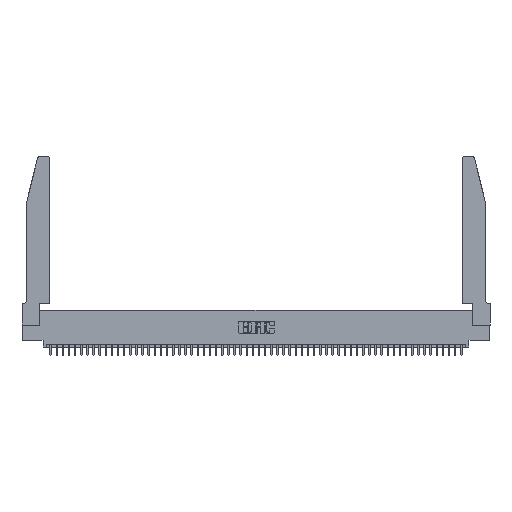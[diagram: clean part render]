
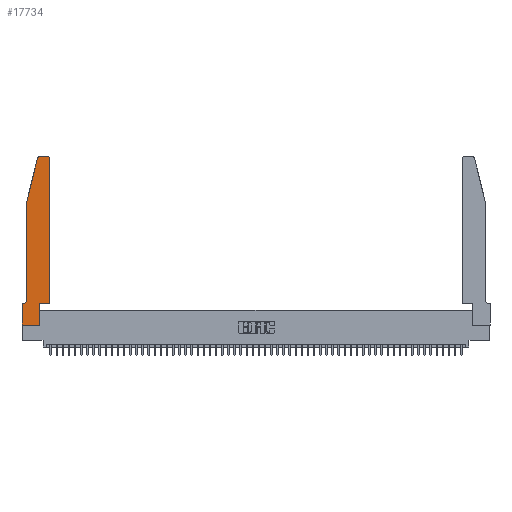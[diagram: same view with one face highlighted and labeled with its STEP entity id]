
A CAD part, top view. The second image highlights one B-rep face of the part: STEP entity #17734.
In plain terms, the highlighted planar face has unit normal (0, 0, 1).
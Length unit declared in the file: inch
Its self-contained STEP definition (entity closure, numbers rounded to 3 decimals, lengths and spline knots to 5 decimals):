
#117 = VERTEX_POINT ( 'NONE', #24283 ) ;
#540 = LINE ( 'NONE', #28226, #33080 ) ;
#622 = DIRECTION ( 'NONE',  ( 1., 0., 0. ) ) ;
#1321 = LINE ( 'NONE', #30457, #33818 ) ;
#1773 = DIRECTION ( 'NONE',  ( 0., 1., 0. ) ) ;
#2243 = CARTESIAN_POINT ( 'NONE',  ( 0.2865, 0.35, 0.37 ) ) ;
#3311 = VERTEX_POINT ( 'NONE', #41952 ) ;
#4764 = AXIS2_PLACEMENT_3D ( 'NONE', #52568, #23818, #53309 ) ;
#4837 = ORIENTED_EDGE ( 'NONE', *, *, #7785, .T. ) ;
#6080 = ORIENTED_EDGE ( 'NONE', *, *, #40368, .T. ) ;
#6818 = EDGE_CURVE ( 'NONE', #35872, #3311, #26489, .T. ) ;
#7785 = EDGE_CURVE ( 'NONE', #3311, #49695, #48779, .T. ) ;
#7859 = VERTEX_POINT ( 'NONE', #28221 ) ;
#7978 = DIRECTION ( 'NONE',  ( 0., 0., 1. ) ) ;
#9416 = ORIENTED_EDGE ( 'NONE', *, *, #14255, .T. ) ;
#9960 = EDGE_CURVE ( 'NONE', #49695, #24837, #51154, .T. ) ;
#10256 = PLANE ( 'NONE',  #4764 ) ;
#10703 = CIRCLE ( 'NONE', #19130, 0.03 ) ;
#10855 = AXIS2_PLACEMENT_3D ( 'NONE', #48891, #23642, #53141 ) ;
#11014 = CARTESIAN_POINT ( 'NONE',  ( 0.4505, 0.35, 0.37 ) ) ;
#11652 = VERTEX_POINT ( 'NONE', #25148 ) ;
#12089 = ORIENTED_EDGE ( 'NONE', *, *, #32029, .T. ) ;
#13085 = CARTESIAN_POINT ( 'NONE',  ( 0.0055, 0.42, 0.37 ) ) ;
#13315 = CARTESIAN_POINT ( 'NONE',  ( 0.4505, 2.72, 0.37 ) ) ;
#14255 = EDGE_CURVE ( 'NONE', #52962, #23506, #51151, .T. ) ;
#15231 = VECTOR ( 'NONE', #622, 39.37008 ) ;
#16194 = VECTOR ( 'NONE', #20317, 39.37008 ) ;
#16230 = CARTESIAN_POINT ( 'NONE',  ( 0.0755, 0.35, 0.37 ) ) ;
#17378 = DIRECTION ( 'NONE',  ( -1., 0., 0. ) ) ;
#17525 = VECTOR ( 'NONE', #19637, 39.37008 ) ;
#17734 = ADVANCED_FACE ( 'NONE', ( #28120 ), #10256, .T. ) ;
#18109 = ORIENTED_EDGE ( 'NONE', *, *, #43499, .T. ) ;
#18536 = CARTESIAN_POINT ( 'NONE',  ( 0.0755, 2., 0.37 ) ) ;
#18870 = VECTOR ( 'NONE', #25044, 39.37008 ) ;
#19130 = AXIS2_PLACEMENT_3D ( 'NONE', #33383, #7978, #37609 ) ;
#19637 = DIRECTION ( 'NONE',  ( 1., 0., 0. ) ) ;
#20111 = ORIENTED_EDGE ( 'NONE', *, *, #31610, .T. ) ;
#20317 = DIRECTION ( 'NONE',  ( -1., 0., 0. ) ) ;
#20764 = CARTESIAN_POINT ( 'NONE',  ( 0.25487, 2.72718, 0.37 ) ) ;
#21594 = CARTESIAN_POINT ( 'NONE',  ( 0., 0., 0.37 ) ) ;
#21973 = DIRECTION ( 'NONE',  ( 0., -1., 0. ) ) ;
#23506 = VERTEX_POINT ( 'NONE', #40249 ) ;
#23642 = DIRECTION ( 'NONE',  ( 0., 0., 1. ) ) ;
#23717 = VECTOR ( 'NONE', #40360, 39.37008 ) ;
#23818 = DIRECTION ( 'NONE',  ( 0., 0., 1. ) ) ;
#24283 = CARTESIAN_POINT ( 'NONE',  ( 0.284, 2.75, 0.37 ) ) ;
#24837 = VERTEX_POINT ( 'NONE', #32240 ) ;
#25044 = DIRECTION ( 'NONE',  ( 0., -1., 0. ) ) ;
#25148 = CARTESIAN_POINT ( 'NONE',  ( 0.0755, 0.42, 0.37 ) ) ;
#26302 = EDGE_CURVE ( 'NONE', #7859, #117, #540, .T. ) ;
#26489 = LINE ( 'NONE', #51314, #15231 ) ;
#26869 = CIRCLE ( 'NONE', #45043, 0.07 ) ;
#27215 = CARTESIAN_POINT ( 'NONE',  ( 0.4505, 0.35, 0.37 ) ) ;
#28120 = FACE_OUTER_BOUND ( 'NONE', #33603, .T. ) ;
#28221 = CARTESIAN_POINT ( 'NONE',  ( 0.4205, 2.75, 0.37 ) ) ;
#28226 = CARTESIAN_POINT ( 'NONE',  ( 0.2605, 2.75, 0.37 ) ) ;
#30098 = LINE ( 'NONE', #41820, #18870 ) ;
#30457 = CARTESIAN_POINT ( 'NONE',  ( 0., 0., 0.37 ) ) ;
#31186 = CARTESIAN_POINT ( 'NONE',  ( 0.0055, 0.35, 0.37 ) ) ;
#31558 = VERTEX_POINT ( 'NONE', #18536 ) ;
#31610 = EDGE_CURVE ( 'NONE', #24837, #47314, #39236, .T. ) ;
#32029 = EDGE_CURVE ( 'NONE', #39002, #31558, #43125, .T. ) ;
#32240 = CARTESIAN_POINT ( 'NONE',  ( 0.4505, 0.35, 0.37 ) ) ;
#32929 = ORIENTED_EDGE ( 'NONE', *, *, #48610, .T. ) ;
#33080 = VECTOR ( 'NONE', #53614, 39.37008 ) ;
#33383 = CARTESIAN_POINT ( 'NONE',  ( 0.4205, 2.72, 0.37 ) ) ;
#33424 = ORIENTED_EDGE ( 'NONE', *, *, #44483, .T. ) ;
#33603 = EDGE_LOOP ( 'NONE', ( #45019, #18109, #12089, #6080, #32929, #9416, #34873, #53192, #4837, #44363, #20111, #33424 ) ) ;
#33818 = VECTOR ( 'NONE', #21973, 39.37008 ) ;
#34873 = ORIENTED_EDGE ( 'NONE', *, *, #52831, .T. ) ;
#35872 = VERTEX_POINT ( 'NONE', #21594 ) ;
#36809 = CARTESIAN_POINT ( 'NONE',  ( 0.2865, 0.35, 0.37 ) ) ;
#37609 = DIRECTION ( 'NONE',  ( 1., 0., 0. ) ) ;
#39002 = VERTEX_POINT ( 'NONE', #20764 ) ;
#39236 = LINE ( 'NONE', #27215, #50412 ) ;
#40249 = CARTESIAN_POINT ( 'NONE',  ( 0., 0.35, 0.37 ) ) ;
#40360 = DIRECTION ( 'NONE',  ( 0., 1., 0. ) ) ;
#40368 = EDGE_CURVE ( 'NONE', #31558, #11652, #30098, .T. ) ;
#40534 = CIRCLE ( 'NONE', #10855, 0.03 ) ;
#41820 = CARTESIAN_POINT ( 'NONE',  ( 0.0755, 2., 0.37 ) ) ;
#41952 = CARTESIAN_POINT ( 'NONE',  ( 0.2865, 0., 0.37 ) ) ;
#42638 = DIRECTION ( 'NONE',  ( 0., 0., -1. ) ) ;
#43125 = LINE ( 'NONE', #46692, #51690 ) ;
#43499 = EDGE_CURVE ( 'NONE', #117, #39002, #40534, .T. ) ;
#44363 = ORIENTED_EDGE ( 'NONE', *, *, #9960, .T. ) ;
#44483 = EDGE_CURVE ( 'NONE', #47314, #7859, #10703, .T. ) ;
#45019 = ORIENTED_EDGE ( 'NONE', *, *, #26302, .T. ) ;
#45043 = AXIS2_PLACEMENT_3D ( 'NONE', #13085, #42638, #17378 ) ;
#46692 = CARTESIAN_POINT ( 'NONE',  ( 0.0755, 2., 0.37 ) ) ;
#47314 = VERTEX_POINT ( 'NONE', #13315 ) ;
#48610 = EDGE_CURVE ( 'NONE', #11652, #52962, #26869, .T. ) ;
#48779 = LINE ( 'NONE', #2243, #23717 ) ;
#48891 = CARTESIAN_POINT ( 'NONE',  ( 0.284, 2.72, 0.37 ) ) ;
#49695 = VERTEX_POINT ( 'NONE', #36809 ) ;
#50412 = VECTOR ( 'NONE', #1773, 39.37008 ) ;
#50906 = DIRECTION ( 'NONE',  ( -0.239, -0.971, 0. ) ) ;
#51151 = LINE ( 'NONE', #16230, #16194 ) ;
#51154 = LINE ( 'NONE', #11014, #17525 ) ;
#51314 = CARTESIAN_POINT ( 'NONE',  ( 0., 0., 0.37 ) ) ;
#51690 = VECTOR ( 'NONE', #50906, 39.37008 ) ;
#52568 = CARTESIAN_POINT ( 'NONE',  ( 0., 0.35, 0.37 ) ) ;
#52831 = EDGE_CURVE ( 'NONE', #23506, #35872, #1321, .T. ) ;
#52962 = VERTEX_POINT ( 'NONE', #31186 ) ;
#53141 = DIRECTION ( 'NONE',  ( 1., 0., 0. ) ) ;
#53192 = ORIENTED_EDGE ( 'NONE', *, *, #6818, .T. ) ;
#53309 = DIRECTION ( 'NONE',  ( 1., 0., 0. ) ) ;
#53614 = DIRECTION ( 'NONE',  ( -1., 0., 0. ) ) ;
